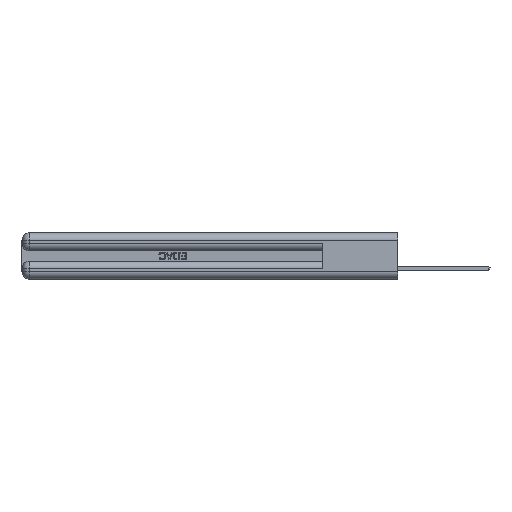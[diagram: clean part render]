
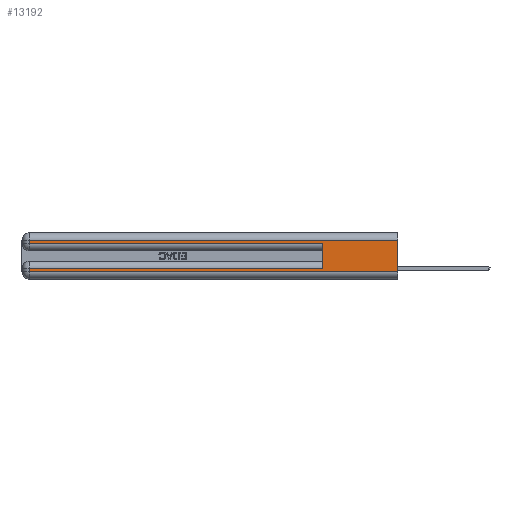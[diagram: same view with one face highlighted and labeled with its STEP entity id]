
A CAD part, left-side view. The second image highlights one B-rep face of the part: STEP entity #13192.
In plain terms, the highlighted planar face has unit normal (-1, 0, 0).
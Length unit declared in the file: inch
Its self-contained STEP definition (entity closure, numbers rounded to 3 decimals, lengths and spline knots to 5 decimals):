
#265 = VECTOR ( 'NONE', #5927, 39.37008 ) ;
#278 = CARTESIAN_POINT ( 'NONE',  ( 0., 0.6, 0.285 ) ) ;
#493 = VERTEX_POINT ( 'NONE', #48424 ) ;
#1388 = CARTESIAN_POINT ( 'NONE',  ( 0., 0., 0.31 ) ) ;
#1943 = CARTESIAN_POINT ( 'NONE',  ( 0., 0., 0.37 ) ) ;
#3209 = VECTOR ( 'NONE', #13527, 39.37008 ) ;
#4732 = ORIENTED_EDGE ( 'NONE', *, *, #44353, .F. ) ;
#4825 = VECTOR ( 'NONE', #36010, 39.37008 ) ;
#4848 = LINE ( 'NONE', #43434, #20089 ) ;
#5927 = DIRECTION ( 'NONE',  ( 0., 0., -1. ) ) ;
#7497 = EDGE_LOOP ( 'NONE', ( #4732, #21847, #47587, #39028, #46544, #14072, #37080, #19152 ) ) ;
#7770 = VECTOR ( 'NONE', #37677, 39.37008 ) ;
#8164 = AXIS2_PLACEMENT_3D ( 'NONE', #18772, #47180, #39350 ) ;
#9268 = CARTESIAN_POINT ( 'NONE',  ( 0., 2.94, 0.37 ) ) ;
#10682 = CARTESIAN_POINT ( 'NONE',  ( 0., 2.94, 0.06 ) ) ;
#11443 = VERTEX_POINT ( 'NONE', #13039 ) ;
#13039 = CARTESIAN_POINT ( 'NONE',  ( 0., 0., 0.31 ) ) ;
#13192 = ADVANCED_FACE ( 'NONE', ( #33453 ), #51106, .F. ) ;
#13197 = EDGE_CURVE ( 'NONE', #45047, #32771, #4848, .T. ) ;
#13527 = DIRECTION ( 'NONE',  ( 0., 0., -1. ) ) ;
#14072 = ORIENTED_EDGE ( 'NONE', *, *, #20800, .T. ) ;
#14145 = LINE ( 'NONE', #9268, #7770 ) ;
#18772 = CARTESIAN_POINT ( 'NONE',  ( 0., 0., 0.37 ) ) ;
#18886 = VERTEX_POINT ( 'NONE', #40614 ) ;
#19125 = DIRECTION ( 'NONE',  ( 0., 0., 1. ) ) ;
#19152 = ORIENTED_EDGE ( 'NONE', *, *, #42406, .T. ) ;
#19886 = VERTEX_POINT ( 'NONE', #10682 ) ;
#20065 = LINE ( 'NONE', #52701, #4825 ) ;
#20089 = VECTOR ( 'NONE', #19125, 39.37008 ) ;
#20800 = EDGE_CURVE ( 'NONE', #45047, #35857, #20065, .T. ) ;
#21153 = DIRECTION ( 'NONE',  ( 0., -1., 0. ) ) ;
#21847 = ORIENTED_EDGE ( 'NONE', *, *, #36640, .T. ) ;
#22469 = CARTESIAN_POINT ( 'NONE',  ( 0., 0.6, 0.085 ) ) ;
#22947 = CARTESIAN_POINT ( 'NONE',  ( 0., 0., 0.06 ) ) ;
#25572 = VECTOR ( 'NONE', #48569, 39.37008 ) ;
#28975 = CARTESIAN_POINT ( 'NONE',  ( 0., 0., 0.06 ) ) ;
#30284 = CARTESIAN_POINT ( 'NONE',  ( 0., 2.94, 0.37 ) ) ;
#32770 = CARTESIAN_POINT ( 'NONE',  ( 0., 0., 0.285 ) ) ;
#32771 = VERTEX_POINT ( 'NONE', #278 ) ;
#33453 = FACE_OUTER_BOUND ( 'NONE', #7497, .T. ) ;
#34283 = VERTEX_POINT ( 'NONE', #22947 ) ;
#35250 = LINE ( 'NONE', #30284, #265 ) ;
#35857 = VERTEX_POINT ( 'NONE', #49617 ) ;
#36010 = DIRECTION ( 'NONE',  ( 0., 1., 0. ) ) ;
#36640 = EDGE_CURVE ( 'NONE', #11443, #18886, #48045, .T. ) ;
#37080 = ORIENTED_EDGE ( 'NONE', *, *, #49670, .T. ) ;
#37677 = DIRECTION ( 'NONE',  ( 0., 0., -1. ) ) ;
#39028 = ORIENTED_EDGE ( 'NONE', *, *, #52262, .T. ) ;
#39350 = DIRECTION ( 'NONE',  ( 0., 0., -1. ) ) ;
#40614 = CARTESIAN_POINT ( 'NONE',  ( 0., 2.94, 0.31 ) ) ;
#42391 = DIRECTION ( 'NONE',  ( 0., 1., 0. ) ) ;
#42406 = EDGE_CURVE ( 'NONE', #19886, #34283, #52350, .T. ) ;
#43434 = CARTESIAN_POINT ( 'NONE',  ( 0., 0.6, 0.145 ) ) ;
#43618 = VECTOR ( 'NONE', #42391, 39.37008 ) ;
#44353 = EDGE_CURVE ( 'NONE', #11443, #34283, #48968, .T. ) ;
#45047 = VERTEX_POINT ( 'NONE', #22469 ) ;
#46544 = ORIENTED_EDGE ( 'NONE', *, *, #13197, .F. ) ;
#47177 = LINE ( 'NONE', #32770, #25572 ) ;
#47180 = DIRECTION ( 'NONE',  ( 1., 0., 0. ) ) ;
#47587 = ORIENTED_EDGE ( 'NONE', *, *, #51096, .T. ) ;
#48045 = LINE ( 'NONE', #1388, #43618 ) ;
#48424 = CARTESIAN_POINT ( 'NONE',  ( 0., 2.94, 0.285 ) ) ;
#48569 = DIRECTION ( 'NONE',  ( 0., -1., 0. ) ) ;
#48968 = LINE ( 'NONE', #1943, #3209 ) ;
#49617 = CARTESIAN_POINT ( 'NONE',  ( 0., 2.94, 0.085 ) ) ;
#49670 = EDGE_CURVE ( 'NONE', #35857, #19886, #14145, .T. ) ;
#51096 = EDGE_CURVE ( 'NONE', #18886, #493, #35250, .T. ) ;
#51106 = PLANE ( 'NONE',  #8164 ) ;
#51746 = VECTOR ( 'NONE', #21153, 39.37008 ) ;
#52262 = EDGE_CURVE ( 'NONE', #493, #32771, #47177, .T. ) ;
#52350 = LINE ( 'NONE', #28975, #51746 ) ;
#52701 = CARTESIAN_POINT ( 'NONE',  ( 0., 0., 0.085 ) ) ;
